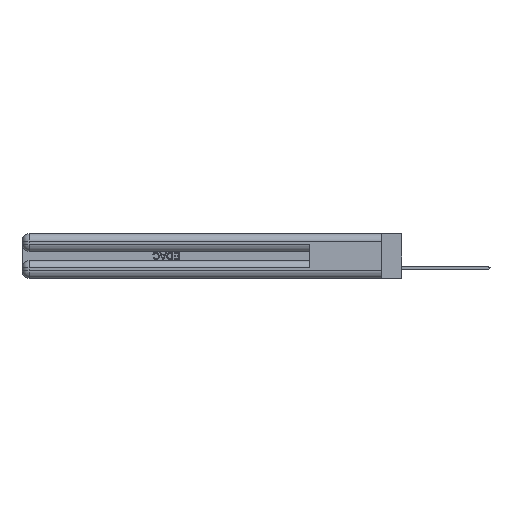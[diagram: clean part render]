
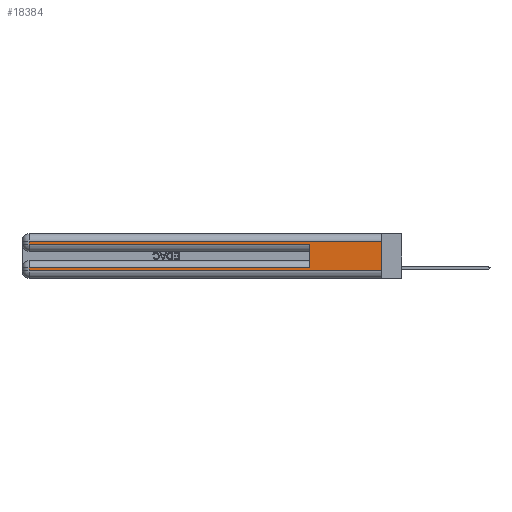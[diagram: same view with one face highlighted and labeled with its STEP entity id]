
A CAD part, left-side view. The second image highlights one B-rep face of the part: STEP entity #18384.
In plain terms, the highlighted planar face has unit normal (-1, 0, 0).
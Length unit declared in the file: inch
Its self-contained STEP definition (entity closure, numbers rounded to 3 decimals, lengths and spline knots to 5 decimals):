
#148 = LINE ( 'NONE', #5122, #13110 ) ;
#2087 = VERTEX_POINT ( 'NONE', #7593 ) ;
#2578 = VECTOR ( 'NONE', #15248, 39.37008 ) ;
#3878 = VECTOR ( 'NONE', #38645, 39.37008 ) ;
#5055 = CARTESIAN_POINT ( 'NONE',  ( 0., 0.6, 0.285 ) ) ;
#5122 = CARTESIAN_POINT ( 'NONE',  ( 0., 2.94, 0.37 ) ) ;
#5694 = CARTESIAN_POINT ( 'NONE',  ( 0., 0., 0.06 ) ) ;
#6055 = ORIENTED_EDGE ( 'NONE', *, *, #30003, .T. ) ;
#6307 = ORIENTED_EDGE ( 'NONE', *, *, #34127, .T. ) ;
#6494 = EDGE_CURVE ( 'NONE', #37042, #16797, #28270, .T. ) ;
#6964 = DIRECTION ( 'NONE',  ( 0., 0., -1. ) ) ;
#7304 = DIRECTION ( 'NONE',  ( 0., 0., 1. ) ) ;
#7593 = CARTESIAN_POINT ( 'NONE',  ( 0., 0.6, 0.085 ) ) ;
#8109 = LINE ( 'NONE', #16040, #22138 ) ;
#8799 = CARTESIAN_POINT ( 'NONE',  ( 0., 0., 0.085 ) ) ;
#10219 = DIRECTION ( 'NONE',  ( 0., 0., -1. ) ) ;
#10661 = VERTEX_POINT ( 'NONE', #5055 ) ;
#11237 = CARTESIAN_POINT ( 'NONE',  ( 0., 0., 0.31 ) ) ;
#11824 = EDGE_CURVE ( 'NONE', #26455, #12195, #41936, .T. ) ;
#12195 = VERTEX_POINT ( 'NONE', #26420 ) ;
#13110 = VECTOR ( 'NONE', #38304, 39.37008 ) ;
#13881 = EDGE_CURVE ( 'NONE', #39631, #12195, #8109, .T. ) ;
#13929 = ORIENTED_EDGE ( 'NONE', *, *, #13881, .F. ) ;
#14014 = CARTESIAN_POINT ( 'NONE',  ( 0., 2.94, 0.31 ) ) ;
#14508 = ORIENTED_EDGE ( 'NONE', *, *, #11824, .T. ) ;
#14599 = VERTEX_POINT ( 'NONE', #16431 ) ;
#14959 = LINE ( 'NONE', #38621, #33075 ) ;
#15248 = DIRECTION ( 'NONE',  ( 0., -1., 0. ) ) ;
#15966 = VECTOR ( 'NONE', #7304, 39.37008 ) ;
#16040 = CARTESIAN_POINT ( 'NONE',  ( 0., 0., 0.37 ) ) ;
#16431 = CARTESIAN_POINT ( 'NONE',  ( 0., 2.94, 0.085 ) ) ;
#16797 = VERTEX_POINT ( 'NONE', #36730 ) ;
#17552 = ORIENTED_EDGE ( 'NONE', *, *, #6494, .T. ) ;
#18384 = ADVANCED_FACE ( 'NONE', ( #35157 ), #23719, .F. ) ;
#18946 = DIRECTION ( 'NONE',  ( 0., 1., 0. ) ) ;
#19951 = CARTESIAN_POINT ( 'NONE',  ( 0., 0.6, 0.145 ) ) ;
#20450 = EDGE_CURVE ( 'NONE', #2087, #10661, #34605, .T. ) ;
#22138 = VECTOR ( 'NONE', #39078, 39.37008 ) ;
#22788 = CARTESIAN_POINT ( 'NONE',  ( 0., 0., 0.285 ) ) ;
#23362 = DIRECTION ( 'NONE',  ( 0., -1., 0. ) ) ;
#23498 = CARTESIAN_POINT ( 'NONE',  ( 0., 2.94, 0.37 ) ) ;
#23719 = PLANE ( 'NONE',  #31171 ) ;
#24059 = VECTOR ( 'NONE', #23362, 39.37008 ) ;
#25688 = LINE ( 'NONE', #8799, #3878 ) ;
#26420 = CARTESIAN_POINT ( 'NONE',  ( 0., 0., 0.06 ) ) ;
#26455 = VERTEX_POINT ( 'NONE', #29928 ) ;
#26900 = CARTESIAN_POINT ( 'NONE',  ( 0., 0., 0.37 ) ) ;
#28270 = LINE ( 'NONE', #23498, #28801 ) ;
#28801 = VECTOR ( 'NONE', #6964, 39.37008 ) ;
#29928 = CARTESIAN_POINT ( 'NONE',  ( 0., 2.94, 0.06 ) ) ;
#30003 = EDGE_CURVE ( 'NONE', #39631, #37042, #14959, .T. ) ;
#30072 = DIRECTION ( 'NONE',  ( 1., 0., 0. ) ) ;
#30270 = EDGE_LOOP ( 'NONE', ( #13929, #6055, #17552, #6307, #37066, #34991, #32768, #14508 ) ) ;
#31171 = AXIS2_PLACEMENT_3D ( 'NONE', #26900, #30072, #10219 ) ;
#32768 = ORIENTED_EDGE ( 'NONE', *, *, #32972, .T. ) ;
#32972 = EDGE_CURVE ( 'NONE', #14599, #26455, #148, .T. ) ;
#33075 = VECTOR ( 'NONE', #18946, 39.37008 ) ;
#34127 = EDGE_CURVE ( 'NONE', #16797, #10661, #34414, .T. ) ;
#34414 = LINE ( 'NONE', #22788, #24059 ) ;
#34605 = LINE ( 'NONE', #19951, #15966 ) ;
#34991 = ORIENTED_EDGE ( 'NONE', *, *, #42768, .T. ) ;
#35157 = FACE_OUTER_BOUND ( 'NONE', #30270, .T. ) ;
#36730 = CARTESIAN_POINT ( 'NONE',  ( 0., 2.94, 0.285 ) ) ;
#37042 = VERTEX_POINT ( 'NONE', #14014 ) ;
#37066 = ORIENTED_EDGE ( 'NONE', *, *, #20450, .F. ) ;
#38304 = DIRECTION ( 'NONE',  ( 0., 0., -1. ) ) ;
#38621 = CARTESIAN_POINT ( 'NONE',  ( 0., 0., 0.31 ) ) ;
#38645 = DIRECTION ( 'NONE',  ( 0., 1., 0. ) ) ;
#39078 = DIRECTION ( 'NONE',  ( 0., 0., -1. ) ) ;
#39631 = VERTEX_POINT ( 'NONE', #11237 ) ;
#41936 = LINE ( 'NONE', #5694, #2578 ) ;
#42768 = EDGE_CURVE ( 'NONE', #2087, #14599, #25688, .T. ) ;
